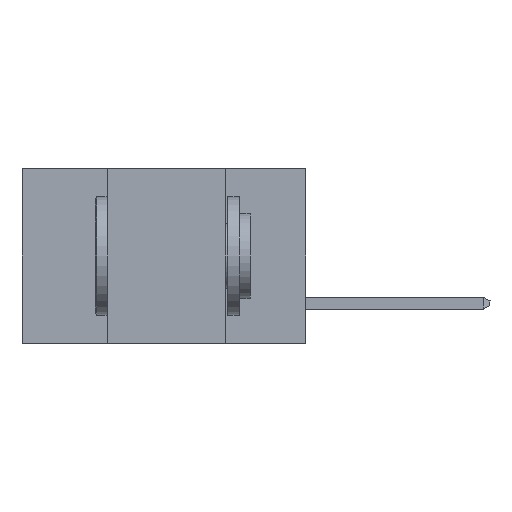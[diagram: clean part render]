
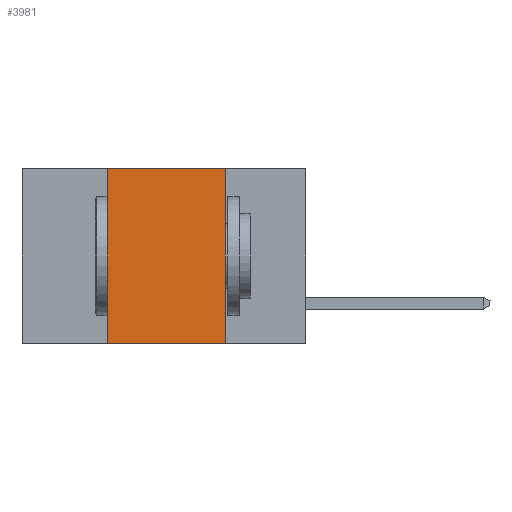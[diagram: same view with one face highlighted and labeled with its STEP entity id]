
A CAD part, left-side view. The second image highlights one B-rep face of the part: STEP entity #3981.
In plain terms, the highlighted planar face has unit normal (-1, 0, 0).
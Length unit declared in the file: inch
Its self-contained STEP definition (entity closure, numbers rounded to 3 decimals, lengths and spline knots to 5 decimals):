
#1094 = EDGE_CURVE ( 'NONE', #23023, #13582, #13837, .T. ) ;
#1193 = CARTESIAN_POINT ( 'NONE',  ( 0., 0.6, 0. ) ) ;
#3183 = CARTESIAN_POINT ( 'NONE',  ( 0., 0.6, 0. ) ) ;
#3981 = ADVANCED_FACE ( 'NONE', ( #13358 ), #19022, .F. ) ;
#4014 = ORIENTED_EDGE ( 'NONE', *, *, #4248, .T. ) ;
#4248 = EDGE_CURVE ( 'NONE', #23237, #13777, #11596, .T. ) ;
#4336 = LINE ( 'NONE', #14668, #27429 ) ;
#6463 = DIRECTION ( 'NONE',  ( 0., -1., 0. ) ) ;
#6470 = AXIS2_PLACEMENT_3D ( 'NONE', #1193, #21372, #16962 ) ;
#7211 = ORIENTED_EDGE ( 'NONE', *, *, #1094, .F. ) ;
#7546 = EDGE_CURVE ( 'NONE', #23237, #23023, #9069, .T. ) ;
#8138 = ORIENTED_EDGE ( 'NONE', *, *, #9975, .F. ) ;
#9069 = LINE ( 'NONE', #28961, #20609 ) ;
#9231 = CARTESIAN_POINT ( 'NONE',  ( 0., 0.17, -0.37 ) ) ;
#9975 = EDGE_CURVE ( 'NONE', #13582, #13777, #4336, .T. ) ;
#10560 = CARTESIAN_POINT ( 'NONE',  ( 0., 0.42, -0.37 ) ) ;
#10865 = CARTESIAN_POINT ( 'NONE',  ( 0., 0.6, -0.37 ) ) ;
#11596 = LINE ( 'NONE', #10865, #16152 ) ;
#13358 = FACE_OUTER_BOUND ( 'NONE', #17690, .T. ) ;
#13582 = VERTEX_POINT ( 'NONE', #25158 ) ;
#13777 = VERTEX_POINT ( 'NONE', #9231 ) ;
#13837 = LINE ( 'NONE', #3183, #27126 ) ;
#14668 = CARTESIAN_POINT ( 'NONE',  ( 0., 0.17, 0. ) ) ;
#15590 = DIRECTION ( 'NONE',  ( 0., 0., 1. ) ) ;
#16152 = VECTOR ( 'NONE', #23544, 39.37008 ) ;
#16962 = DIRECTION ( 'NONE',  ( 0., 0., -1. ) ) ;
#17690 = EDGE_LOOP ( 'NONE', ( #8138, #7211, #23346, #4014 ) ) ;
#19022 = PLANE ( 'NONE',  #6470 ) ;
#20609 = VECTOR ( 'NONE', #15590, 39.37008 ) ;
#21372 = DIRECTION ( 'NONE',  ( 1., 0., 0. ) ) ;
#23023 = VERTEX_POINT ( 'NONE', #25014 ) ;
#23237 = VERTEX_POINT ( 'NONE', #10560 ) ;
#23346 = ORIENTED_EDGE ( 'NONE', *, *, #7546, .F. ) ;
#23544 = DIRECTION ( 'NONE',  ( 0., -1., 0. ) ) ;
#23744 = DIRECTION ( 'NONE',  ( 0., 0., -1. ) ) ;
#25014 = CARTESIAN_POINT ( 'NONE',  ( 0., 0.42, 0. ) ) ;
#25158 = CARTESIAN_POINT ( 'NONE',  ( 0., 0.17, 0. ) ) ;
#27126 = VECTOR ( 'NONE', #6463, 39.37008 ) ;
#27429 = VECTOR ( 'NONE', #23744, 39.37008 ) ;
#28961 = CARTESIAN_POINT ( 'NONE',  ( 0., 0.42, 0. ) ) ;
